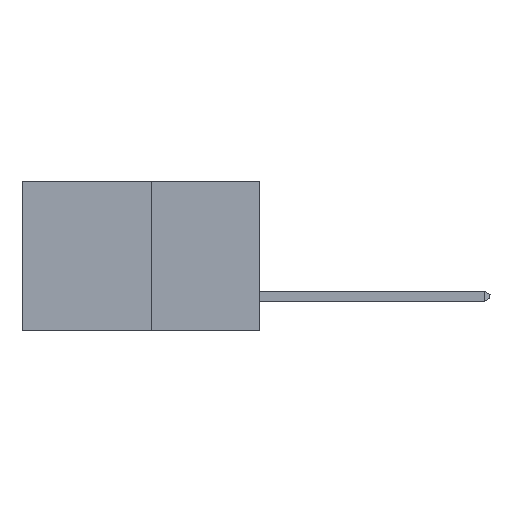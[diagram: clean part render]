
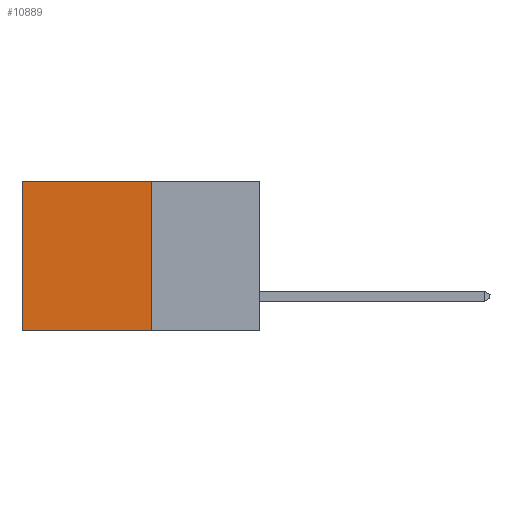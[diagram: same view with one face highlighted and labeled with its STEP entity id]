
A CAD part, left-side view. The second image highlights one B-rep face of the part: STEP entity #10889.
In plain terms, the highlighted planar face has unit normal (-1, 0, 0).
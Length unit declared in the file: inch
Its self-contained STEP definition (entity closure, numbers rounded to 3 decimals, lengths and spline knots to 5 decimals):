
#52 = CARTESIAN_POINT ( 'NONE',  ( 0.277, 0.27, -0.37 ) ) ;
#242 = ORIENTED_EDGE ( 'NONE', *, *, #12986, .F. ) ;
#1103 = VECTOR ( 'NONE', #9804, 39.37008 ) ;
#2243 = DIRECTION ( 'NONE',  ( 0., 0., -1. ) ) ;
#3757 = LINE ( 'NONE', #52, #14630 ) ;
#5447 = CARTESIAN_POINT ( 'NONE',  ( 0.277, 0.27, 0. ) ) ;
#5835 = CARTESIAN_POINT ( 'NONE',  ( 0.277, 0.27, 0. ) ) ;
#6551 = VERTEX_POINT ( 'NONE', #5835 ) ;
#7622 = EDGE_LOOP ( 'NONE', ( #8982, #242, #18254, #8942 ) ) ;
#7656 = CARTESIAN_POINT ( 'NONE',  ( 0.277, 0.27, -0.37 ) ) ;
#8594 = AXIS2_PLACEMENT_3D ( 'NONE', #15733, #22214, #9243 ) ;
#8942 = ORIENTED_EDGE ( 'NONE', *, *, #19773, .T. ) ;
#8982 = ORIENTED_EDGE ( 'NONE', *, *, #21560, .T. ) ;
#9243 = DIRECTION ( 'NONE',  ( 0., 0., -1. ) ) ;
#9483 = EDGE_CURVE ( 'NONE', #6551, #22499, #3757, .T. ) ;
#9804 = DIRECTION ( 'NONE',  ( 0., 1., 0. ) ) ;
#10586 = DIRECTION ( 'NONE',  ( 0., 0., -1. ) ) ;
#10889 = ADVANCED_FACE ( 'NONE', ( #17580 ), #20057, .F. ) ;
#11649 = VECTOR ( 'NONE', #20571, 39.37008 ) ;
#12627 = CARTESIAN_POINT ( 'NONE',  ( 0.277, 0.59, 0. ) ) ;
#12986 = EDGE_CURVE ( 'NONE', #22499, #13675, #18376, .T. ) ;
#13675 = VERTEX_POINT ( 'NONE', #14484 ) ;
#14314 = LINE ( 'NONE', #19220, #20024 ) ;
#14484 = CARTESIAN_POINT ( 'NONE',  ( 0.277, 0.59, -0.37 ) ) ;
#14630 = VECTOR ( 'NONE', #2243, 39.37008 ) ;
#15733 = CARTESIAN_POINT ( 'NONE',  ( 0.277, 0.27, -0.37 ) ) ;
#16750 = LINE ( 'NONE', #5447, #11649 ) ;
#17580 = FACE_OUTER_BOUND ( 'NONE', #7622, .T. ) ;
#18254 = ORIENTED_EDGE ( 'NONE', *, *, #9483, .F. ) ;
#18376 = LINE ( 'NONE', #7656, #1103 ) ;
#19220 = CARTESIAN_POINT ( 'NONE',  ( 0.277, 0.59, -0.37 ) ) ;
#19773 = EDGE_CURVE ( 'NONE', #6551, #20517, #16750, .T. ) ;
#20024 = VECTOR ( 'NONE', #10586, 39.37008 ) ;
#20057 = PLANE ( 'NONE',  #8594 ) ;
#20517 = VERTEX_POINT ( 'NONE', #12627 ) ;
#20571 = DIRECTION ( 'NONE',  ( 0., 1., 0. ) ) ;
#21560 = EDGE_CURVE ( 'NONE', #20517, #13675, #14314, .T. ) ;
#22214 = DIRECTION ( 'NONE',  ( 1., 0., 0. ) ) ;
#22499 = VERTEX_POINT ( 'NONE', #24335 ) ;
#24335 = CARTESIAN_POINT ( 'NONE',  ( 0.277, 0.27, -0.37 ) ) ;
